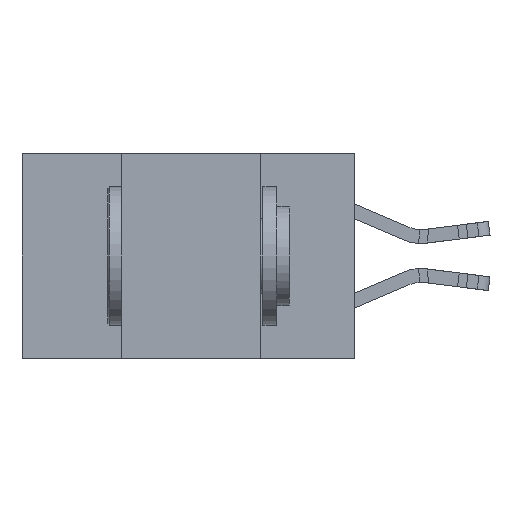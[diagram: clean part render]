
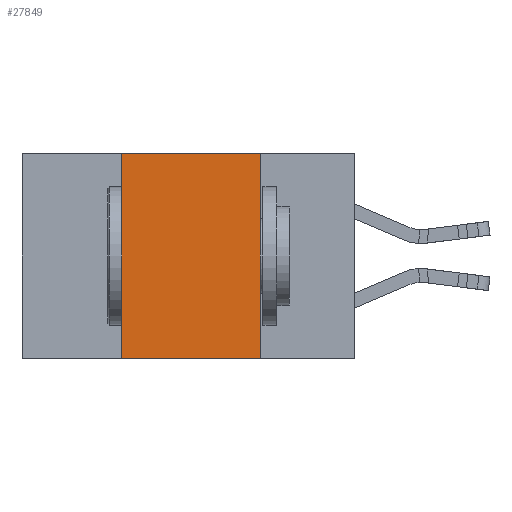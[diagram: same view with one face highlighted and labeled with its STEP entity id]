
A CAD part, left-side view. The second image highlights one B-rep face of the part: STEP entity #27849.
In plain terms, the highlighted planar face has unit normal (-1, 0, 0).
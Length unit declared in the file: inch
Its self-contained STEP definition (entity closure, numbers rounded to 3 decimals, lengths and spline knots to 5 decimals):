
#171 = EDGE_CURVE ( 'NONE', #8305, #4671, #25587, .T. ) ;
#1000 = DIRECTION ( 'NONE',  ( 0., 0., -1. ) ) ;
#1789 = VERTEX_POINT ( 'NONE', #16775 ) ;
#2554 = EDGE_CURVE ( 'NONE', #1789, #10732, #24271, .T. ) ;
#3579 = EDGE_LOOP ( 'NONE', ( #4623, #9183, #11697, #25434 ) ) ;
#4623 = ORIENTED_EDGE ( 'NONE', *, *, #14381, .F. ) ;
#4671 = VERTEX_POINT ( 'NONE', #23114 ) ;
#5264 = DIRECTION ( 'NONE',  ( 1., 0., 0. ) ) ;
#6124 = CARTESIAN_POINT ( 'NONE',  ( 0., 0.42, 0. ) ) ;
#6856 = EDGE_CURVE ( 'NONE', #1789, #8305, #9879, .T. ) ;
#8305 = VERTEX_POINT ( 'NONE', #27330 ) ;
#8686 = LINE ( 'NONE', #14583, #15453 ) ;
#9183 = ORIENTED_EDGE ( 'NONE', *, *, #171, .F. ) ;
#9879 = LINE ( 'NONE', #6124, #21217 ) ;
#10405 = CARTESIAN_POINT ( 'NONE',  ( 0., 0.6, 0. ) ) ;
#10732 = VERTEX_POINT ( 'NONE', #15829 ) ;
#10826 = DIRECTION ( 'NONE',  ( 0., 0., 1. ) ) ;
#11697 = ORIENTED_EDGE ( 'NONE', *, *, #6856, .F. ) ;
#12266 = VECTOR ( 'NONE', #18065, 39.37008 ) ;
#14381 = EDGE_CURVE ( 'NONE', #4671, #10732, #8686, .T. ) ;
#14583 = CARTESIAN_POINT ( 'NONE',  ( 0., 0.17, 0. ) ) ;
#15453 = VECTOR ( 'NONE', #1000, 39.37008 ) ;
#15829 = CARTESIAN_POINT ( 'NONE',  ( 0., 0.17, -0.37 ) ) ;
#16775 = CARTESIAN_POINT ( 'NONE',  ( 0., 0.42, -0.37 ) ) ;
#18059 = FACE_OUTER_BOUND ( 'NONE', #3579, .T. ) ;
#18065 = DIRECTION ( 'NONE',  ( 0., -1., 0. ) ) ;
#18090 = CARTESIAN_POINT ( 'NONE',  ( 0., 0.6, -0.37 ) ) ;
#18799 = CARTESIAN_POINT ( 'NONE',  ( 0., 0.6, 0. ) ) ;
#19649 = VECTOR ( 'NONE', #25233, 39.37008 ) ;
#21045 = DIRECTION ( 'NONE',  ( 0., 0., -1. ) ) ;
#21217 = VECTOR ( 'NONE', #10826, 39.37008 ) ;
#23114 = CARTESIAN_POINT ( 'NONE',  ( 0., 0.17, 0. ) ) ;
#23205 = PLANE ( 'NONE',  #27241 ) ;
#24271 = LINE ( 'NONE', #18090, #12266 ) ;
#25233 = DIRECTION ( 'NONE',  ( 0., -1., 0. ) ) ;
#25434 = ORIENTED_EDGE ( 'NONE', *, *, #2554, .T. ) ;
#25587 = LINE ( 'NONE', #10405, #19649 ) ;
#27241 = AXIS2_PLACEMENT_3D ( 'NONE', #18799, #5264, #21045 ) ;
#27330 = CARTESIAN_POINT ( 'NONE',  ( 0., 0.42, 0. ) ) ;
#27849 = ADVANCED_FACE ( 'NONE', ( #18059 ), #23205, .F. ) ;
